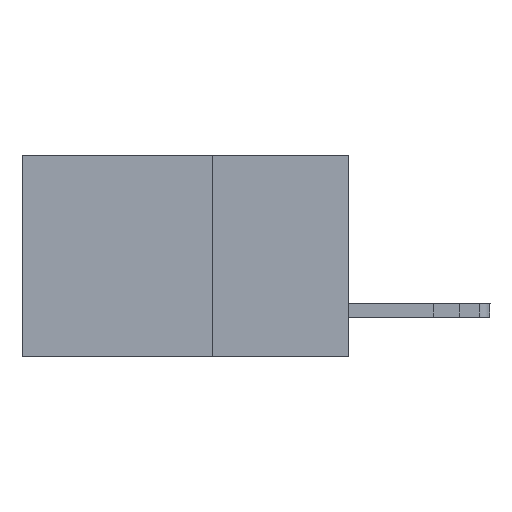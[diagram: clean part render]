
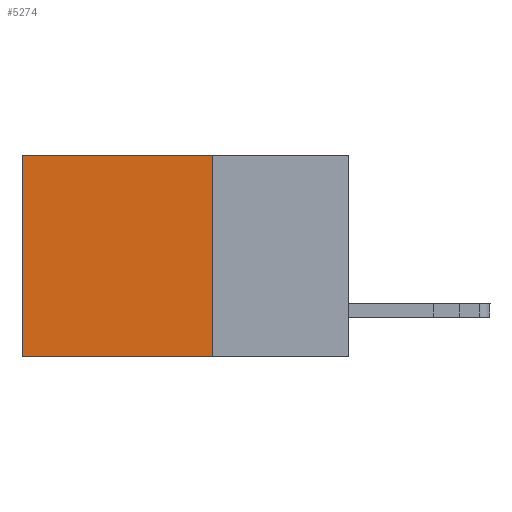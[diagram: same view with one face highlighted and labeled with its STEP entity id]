
A CAD part, left-side view. The second image highlights one B-rep face of the part: STEP entity #5274.
In plain terms, the highlighted planar face has unit normal (-1, 0, 0).
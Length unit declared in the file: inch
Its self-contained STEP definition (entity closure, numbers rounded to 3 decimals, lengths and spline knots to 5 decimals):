
#38 = ORIENTED_EDGE ( 'NONE', *, *, #8688, .T. ) ;
#534 = EDGE_CURVE ( 'NONE', #2086, #9746, #10004, .T. ) ;
#609 = CARTESIAN_POINT ( 'NONE',  ( 0.298, 0.25, 0. ) ) ;
#669 = CARTESIAN_POINT ( 'NONE',  ( 0.298, 0.25, 0. ) ) ;
#2086 = VERTEX_POINT ( 'NONE', #669 ) ;
#2656 = FACE_OUTER_BOUND ( 'NONE', #10886, .T. ) ;
#3040 = ORIENTED_EDGE ( 'NONE', *, *, #534, .F. ) ;
#3068 = VERTEX_POINT ( 'NONE', #6248 ) ;
#3797 = LINE ( 'NONE', #10374, #11604 ) ;
#4108 = VECTOR ( 'NONE', #8534, 39.37008 ) ;
#4454 = DIRECTION ( 'NONE',  ( 0., 0., -1. ) ) ;
#4459 = VECTOR ( 'NONE', #11026, 39.37008 ) ;
#4575 = CARTESIAN_POINT ( 'NONE',  ( 0.298, 0.25, -0.37 ) ) ;
#4593 = DIRECTION ( 'NONE',  ( 1., 0., 0. ) ) ;
#4671 = LINE ( 'NONE', #609, #5593 ) ;
#5155 = ORIENTED_EDGE ( 'NONE', *, *, #8262, .F. ) ;
#5274 = ADVANCED_FACE ( 'NONE', ( #2656 ), #10437, .F. ) ;
#5366 = ORIENTED_EDGE ( 'NONE', *, *, #12681, .T. ) ;
#5593 = VECTOR ( 'NONE', #8579, 39.37008 ) ;
#5627 = CARTESIAN_POINT ( 'NONE',  ( 0.298, 0.6, 0. ) ) ;
#5650 = DIRECTION ( 'NONE',  ( 0., 0., -1. ) ) ;
#6248 = CARTESIAN_POINT ( 'NONE',  ( 0.298, 0.6, -0.37 ) ) ;
#7191 = AXIS2_PLACEMENT_3D ( 'NONE', #11353, #4593, #4454 ) ;
#8228 = CARTESIAN_POINT ( 'NONE',  ( 0.298, 0.25, 0. ) ) ;
#8262 = EDGE_CURVE ( 'NONE', #9746, #3068, #12378, .T. ) ;
#8534 = DIRECTION ( 'NONE',  ( 0., 1., 0. ) ) ;
#8579 = DIRECTION ( 'NONE',  ( 0., 1., 0. ) ) ;
#8688 = EDGE_CURVE ( 'NONE', #10016, #3068, #3797, .T. ) ;
#9746 = VERTEX_POINT ( 'NONE', #11781 ) ;
#10004 = LINE ( 'NONE', #8228, #4459 ) ;
#10016 = VERTEX_POINT ( 'NONE', #5627 ) ;
#10374 = CARTESIAN_POINT ( 'NONE',  ( 0.298, 0.6, 0. ) ) ;
#10437 = PLANE ( 'NONE',  #7191 ) ;
#10886 = EDGE_LOOP ( 'NONE', ( #38, #5155, #3040, #5366 ) ) ;
#11026 = DIRECTION ( 'NONE',  ( 0., 0., -1. ) ) ;
#11353 = CARTESIAN_POINT ( 'NONE',  ( 0.298, 0.25, 0. ) ) ;
#11604 = VECTOR ( 'NONE', #5650, 39.37008 ) ;
#11781 = CARTESIAN_POINT ( 'NONE',  ( 0.298, 0.25, -0.37 ) ) ;
#12378 = LINE ( 'NONE', #4575, #4108 ) ;
#12681 = EDGE_CURVE ( 'NONE', #2086, #10016, #4671, .T. ) ;
